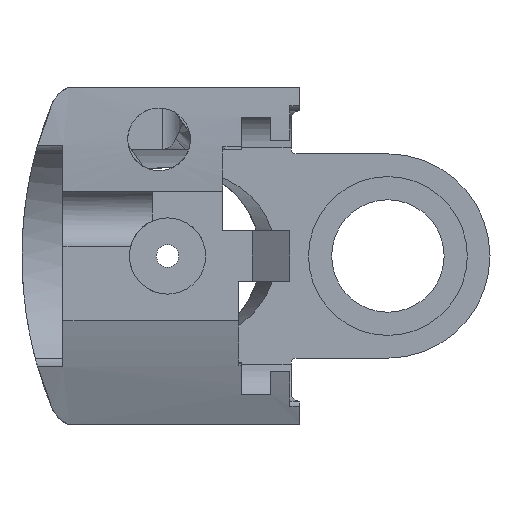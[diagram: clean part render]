
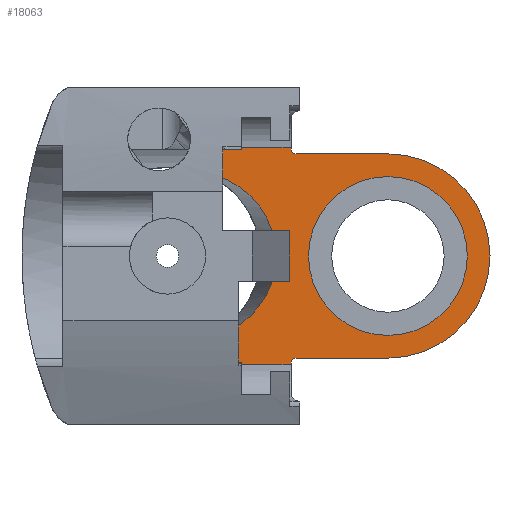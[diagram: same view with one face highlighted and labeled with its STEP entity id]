
A CAD part, left-side view. The second image highlights one B-rep face of the part: STEP entity #18063.
In plain terms, the highlighted planar face has unit normal (-1, 0, 0).
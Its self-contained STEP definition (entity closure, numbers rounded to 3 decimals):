
#108 = VERTEX_POINT ( 'NONE', #15725 ) ;
#186 = ORIENTED_EDGE ( 'NONE', *, *, #3920, .T. ) ;
#211 = VERTEX_POINT ( 'NONE', #18228 ) ;
#392 = AXIS2_PLACEMENT_3D ( 'NONE', #1349, #14642, #3253 ) ;
#750 = LINE ( 'NONE', #20041, #20405 ) ;
#933 = EDGE_CURVE ( 'NONE', #13827, #10481, #3043, .T. ) ;
#980 = CARTESIAN_POINT ( 'NONE',  ( 70.663, -18.028, 0. ) ) ;
#1235 = CARTESIAN_POINT ( 'NONE',  ( 70.663, -11.024, -8.109 ) ) ;
#1349 = CARTESIAN_POINT ( 'NONE',  ( 70.663, -10.735, 8.506 ) ) ;
#1672 = VERTEX_POINT ( 'NONE', #8941 ) ;
#1730 = VECTOR ( 'NONE', #19541, 1000. ) ;
#2362 = DIRECTION ( 'NONE',  ( -1., 0., 0. ) ) ;
#2439 = ORIENTED_EDGE ( 'NONE', *, *, #2717, .F. ) ;
#2464 = CARTESIAN_POINT ( 'NONE',  ( 70.663, -10.735, -8.506 ) ) ;
#2717 = EDGE_CURVE ( 'NONE', #21303, #7650, #23750, .T. ) ;
#2771 = ORIENTED_EDGE ( 'NONE', *, *, #11736, .T. ) ;
#2812 = CARTESIAN_POINT ( 'NONE',  ( 70.663, -11.024, 8.109 ) ) ;
#2880 = DIRECTION ( 'NONE',  ( 0., 0., -1. ) ) ;
#3043 =( BOUNDED_CURVE ( )  B_SPLINE_CURVE ( 3, ( #4306, #15705, #17612, #6243 ),
 .UNSPECIFIED., .F., .F. ) 
 B_SPLINE_CURVE_WITH_KNOTS ( ( 4, 4 ),
 ( 1.861, 4.422 ),
 .UNSPECIFIED. ) 
 CURVE ( )  GEOMETRIC_REPRESENTATION_ITEM ( )  RATIONAL_B_SPLINE_CURVE ( ( 1., 0.524, 0.524, 1. ) ) 
 REPRESENTATION_ITEM ( '' )  );
#3253 = DIRECTION ( 'NONE',  ( 0., 0.707, -0.707 ) ) ;
#3455 = DIRECTION ( 'NONE',  ( 0., 0., 1. ) ) ;
#3559 = CARTESIAN_POINT ( 'NONE',  ( 70.663, -18.028, 8.109 ) ) ;
#3731 = CARTESIAN_POINT ( 'NONE',  ( 70.663, -10.338, 8.649 ) ) ;
#3920 = EDGE_CURVE ( 'NONE', #21886, #1672, #13053, .T. ) ;
#4205 = DIRECTION ( 'NONE',  ( 0., 0., -1. ) ) ;
#4306 = CARTESIAN_POINT ( 'NONE',  ( 70.663, -4.204, 6.456 ) ) ;
#4310 = CIRCLE ( 'NONE', #8983, 0.397 ) ;
#4313 = CARTESIAN_POINT ( 'NONE',  ( 70.663, -11.024, -8.649 ) ) ;
#4382 = DIRECTION ( 'NONE',  ( 0., 0.707, 0.707 ) ) ;
#4461 = AXIS2_PLACEMENT_3D ( 'NONE', #18674, #7294, #20577 ) ;
#4467 = CARTESIAN_POINT ( 'NONE',  ( 70.663, -4.204, -8.649 ) ) ;
#4654 = DIRECTION ( 'NONE',  ( 0., 1., 0. ) ) ;
#5397 = ORIENTED_EDGE ( 'NONE', *, *, #15317, .T. ) ;
#5918 = AXIS2_PLACEMENT_3D ( 'NONE', #2464, #15784, #4382 ) ;
#5969 = VERTEX_POINT ( 'NONE', #19089 ) ;
#6243 = CARTESIAN_POINT ( 'NONE',  ( 70.663, -4.204, -6.456 ) ) ;
#6419 = VECTOR ( 'NONE', #20284, 1000. ) ;
#6461 = CARTESIAN_POINT ( 'NONE',  ( 70.663, -10.454, -8.225 ) ) ;
#6987 = CARTESIAN_POINT ( 'NONE',  ( 70.663, -10.735, 8.506 ) ) ;
#7013 = LINE ( 'NONE', #1235, #6419 ) ;
#7152 = EDGE_CURVE ( 'NONE', #5969, #24042, #10373, .T. ) ;
#7294 = DIRECTION ( 'NONE',  ( 1., 0., 0. ) ) ;
#7617 = ORIENTED_EDGE ( 'NONE', *, *, #7152, .T. ) ;
#7650 = VERTEX_POINT ( 'NONE', #6461 ) ;
#7992 = LINE ( 'NONE', #4313, #1730 ) ;
#8511 = ORIENTED_EDGE ( 'NONE', *, *, #23953, .T. ) ;
#8721 = ORIENTED_EDGE ( 'NONE', *, *, #11342, .T. ) ;
#8742 = VECTOR ( 'NONE', #4654, 1000. ) ;
#8877 = DIRECTION ( 'NONE',  ( 0., 0.707, -0.707 ) ) ;
#8941 = CARTESIAN_POINT ( 'NONE',  ( 70.663, -18.028, 6.306 ) ) ;
#8983 = AXIS2_PLACEMENT_3D ( 'NONE', #13776, #2362, #15688 ) ;
#9155 = CARTESIAN_POINT ( 'NONE',  ( 70.663, -18.028, 0. ) ) ;
#9309 = CARTESIAN_POINT ( 'NONE',  ( 70.663, -10.338, 9.053 ) ) ;
#9490 = VERTEX_POINT ( 'NONE', #13980 ) ;
#9735 = ORIENTED_EDGE ( 'NONE', *, *, #13936, .F. ) ;
#9830 = CARTESIAN_POINT ( 'NONE',  ( 70.663, -10.338, -8.649 ) ) ;
#10022 = ORIENTED_EDGE ( 'NONE', *, *, #13080, .T. ) ;
#10174 = ORIENTED_EDGE ( 'NONE', *, *, #933, .T. ) ;
#10373 = CIRCLE ( 'NONE', #20545, 8.109 ) ;
#10382 = EDGE_CURVE ( 'NONE', #23669, #18039, #21201, .T. ) ;
#10473 = VECTOR ( 'NONE', #3455, 1000. ) ;
#10481 = VERTEX_POINT ( 'NONE', #22723 ) ;
#11066 = DIRECTION ( 'NONE',  ( 0., 0., -1. ) ) ;
#11342 = EDGE_CURVE ( 'NONE', #10481, #108, #13420, .T. ) ;
#11736 = EDGE_CURVE ( 'NONE', #1672, #21886, #22207, .T. ) ;
#11757 = ORIENTED_EDGE ( 'NONE', *, *, #14888, .T. ) ;
#12147 = AXIS2_PLACEMENT_3D ( 'NONE', #6987, #20270, #8877 ) ;
#12218 = EDGE_CURVE ( 'NONE', #19275, #211, #17742, .T. ) ;
#12240 = CARTESIAN_POINT ( 'NONE',  ( 70.663, -4.204, 6.456 ) ) ;
#12325 = EDGE_LOOP ( 'NONE', ( #17661, #13889, #2439, #8511, #7617, #5397, #14896, #9735, #10022, #11757, #18272, #10174, #8721, #19150 ) ) ;
#12952 = VECTOR ( 'NONE', #20697, 1000. ) ;
#13053 = CIRCLE ( 'NONE', #4461, 6.306 ) ;
#13080 = EDGE_CURVE ( 'NONE', #9490, #19401, #23044, .T. ) ;
#13420 = LINE ( 'NONE', #4467, #19079 ) ;
#13776 = CARTESIAN_POINT ( 'NONE',  ( 70.663, -10.735, -8.506 ) ) ;
#13792 = VERTEX_POINT ( 'NONE', #19747 ) ;
#13827 = VERTEX_POINT ( 'NONE', #12240 ) ;
#13889 = ORIENTED_EDGE ( 'NONE', *, *, #22175, .F. ) ;
#13936 = EDGE_CURVE ( 'NONE', #9490, #19275, #20952, .T. ) ;
#13966 = CARTESIAN_POINT ( 'NONE',  ( 70.663, -10.735, -8.109 ) ) ;
#13980 = CARTESIAN_POINT ( 'NONE',  ( 70.663, -10.338, 8.506 ) ) ;
#14276 = DIRECTION ( 'NONE',  ( -1., 0., 0. ) ) ;
#14642 = DIRECTION ( 'NONE',  ( -1., 0., 0. ) ) ;
#14649 = CARTESIAN_POINT ( 'NONE',  ( 70.663, -11.024, 8.649 ) ) ;
#14753 = CARTESIAN_POINT ( 'NONE',  ( 70.663, -10.338, -0.944 ) ) ;
#14888 = EDGE_CURVE ( 'NONE', #19401, #13792, #20293, .T. ) ;
#14896 = ORIENTED_EDGE ( 'NONE', *, *, #12218, .F. ) ;
#15317 = EDGE_CURVE ( 'NONE', #24042, #211, #23292, .T. ) ;
#15612 = DIRECTION ( 'NONE',  ( -1., 0., 0. ) ) ;
#15688 = DIRECTION ( 'NONE',  ( 0., 0.707, 0.707 ) ) ;
#15705 = CARTESIAN_POINT ( 'NONE',  ( 70.663, -12.296, 4.104 ) ) ;
#15725 = CARTESIAN_POINT ( 'NONE',  ( 70.663, -4.204, -8.649 ) ) ;
#15784 = DIRECTION ( 'NONE',  ( -1., 0., 0. ) ) ;
#17366 = CARTESIAN_POINT ( 'NONE',  ( 70.663, -10.338, -8.506 ) ) ;
#17552 = FACE_BOUND ( 'NONE', #23006, .T. ) ;
#17612 = CARTESIAN_POINT ( 'NONE',  ( 70.663, -12.296, -4.104 ) ) ;
#17661 = ORIENTED_EDGE ( 'NONE', *, *, #10382, .T. ) ;
#17742 = CIRCLE ( 'NONE', #12147, 0.397 ) ;
#17791 = DIRECTION ( 'NONE',  ( 0., 0., -1. ) ) ;
#18039 = VERTEX_POINT ( 'NONE', #17366 ) ;
#18063 = ADVANCED_FACE ( 'NONE', ( #21983, #17552 ), #23136, .T. ) ;
#18127 = DIRECTION ( 'NONE',  ( 0., 0., -1. ) ) ;
#18228 = CARTESIAN_POINT ( 'NONE',  ( 70.663, -10.735, 8.109 ) ) ;
#18272 = ORIENTED_EDGE ( 'NONE', *, *, #21844, .T. ) ;
#18300 = CARTESIAN_POINT ( 'NONE',  ( 70.663, -18.028, -6.306 ) ) ;
#18582 = DIRECTION ( 'NONE',  ( 0., 1., 0. ) ) ;
#18674 = CARTESIAN_POINT ( 'NONE',  ( 70.663, -18.028, 0. ) ) ;
#19079 = VECTOR ( 'NONE', #17791, 1000. ) ;
#19089 = CARTESIAN_POINT ( 'NONE',  ( 70.663, -18.028, -8.109 ) ) ;
#19150 = ORIENTED_EDGE ( 'NONE', *, *, #19177, .F. ) ;
#19177 = EDGE_CURVE ( 'NONE', #23669, #108, #7992, .T. ) ;
#19275 = VERTEX_POINT ( 'NONE', #23971 ) ;
#19401 = VERTEX_POINT ( 'NONE', #3731 ) ;
#19541 = DIRECTION ( 'NONE',  ( 0., 1., 0. ) ) ;
#19697 = VECTOR ( 'NONE', #18582, 1000. ) ;
#19747 = CARTESIAN_POINT ( 'NONE',  ( 70.663, -4.204, 8.649 ) ) ;
#20041 = CARTESIAN_POINT ( 'NONE',  ( 70.663, -4.204, -8.649 ) ) ;
#20270 = DIRECTION ( 'NONE',  ( -1., 0., 0. ) ) ;
#20284 = DIRECTION ( 'NONE',  ( 0., -1., 0. ) ) ;
#20293 = LINE ( 'NONE', #14649, #19697 ) ;
#20405 = VECTOR ( 'NONE', #18127, 1000. ) ;
#20545 = AXIS2_PLACEMENT_3D ( 'NONE', #980, #14276, #2880 ) ;
#20577 = DIRECTION ( 'NONE',  ( 0., 0., -1. ) ) ;
#20697 = DIRECTION ( 'NONE',  ( 0., 0., 1. ) ) ;
#20952 = CIRCLE ( 'NONE', #392, 0.397 ) ;
#21178 = CARTESIAN_POINT ( 'NONE',  ( 70.663, -11.024, 8.109 ) ) ;
#21201 = LINE ( 'NONE', #14753, #10473 ) ;
#21303 = VERTEX_POINT ( 'NONE', #13966 ) ;
#21844 = EDGE_CURVE ( 'NONE', #13792, #13827, #750, .T. ) ;
#21886 = VERTEX_POINT ( 'NONE', #18300 ) ;
#21983 = FACE_OUTER_BOUND ( 'NONE', #12325, .T. ) ;
#22175 = EDGE_CURVE ( 'NONE', #7650, #18039, #4310, .T. ) ;
#22207 = CIRCLE ( 'NONE', #23280, 6.306 ) ;
#22444 = DIRECTION ( 'NONE',  ( 1., 0., 0. ) ) ;
#22723 = CARTESIAN_POINT ( 'NONE',  ( 70.663, -4.204, -6.456 ) ) ;
#23006 = EDGE_LOOP ( 'NONE', ( #186, #2771 ) ) ;
#23044 = LINE ( 'NONE', #9309, #12952 ) ;
#23136 = PLANE ( 'NONE',  #24004 ) ;
#23280 = AXIS2_PLACEMENT_3D ( 'NONE', #9155, #22444, #11066 ) ;
#23292 = LINE ( 'NONE', #2812, #8742 ) ;
#23669 = VERTEX_POINT ( 'NONE', #9830 ) ;
#23750 = CIRCLE ( 'NONE', #5918, 0.397 ) ;
#23953 = EDGE_CURVE ( 'NONE', #21303, #5969, #7013, .T. ) ;
#23971 = CARTESIAN_POINT ( 'NONE',  ( 70.663, -10.454, 8.225 ) ) ;
#24004 = AXIS2_PLACEMENT_3D ( 'NONE', #21178, #15612, #4205 ) ;
#24042 = VERTEX_POINT ( 'NONE', #3559 ) ;
